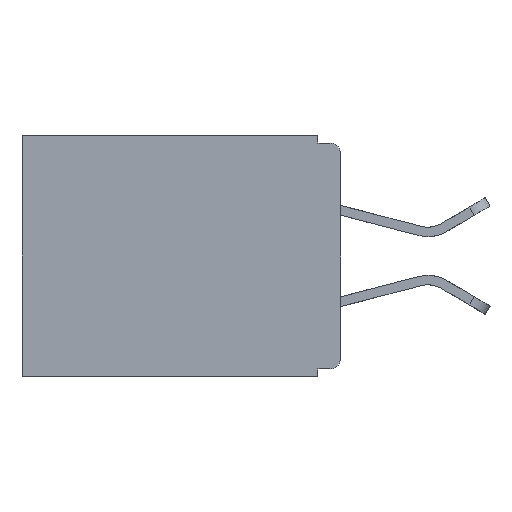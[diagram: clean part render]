
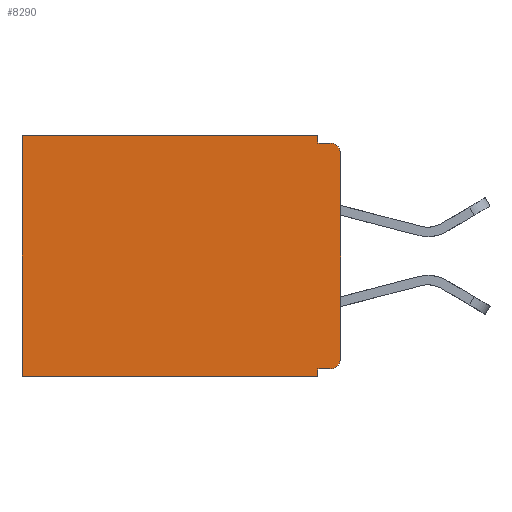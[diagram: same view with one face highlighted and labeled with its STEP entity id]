
A CAD part, left-side view. The second image highlights one B-rep face of the part: STEP entity #8290.
In plain terms, the highlighted planar face has unit normal (-1, 0, 0).
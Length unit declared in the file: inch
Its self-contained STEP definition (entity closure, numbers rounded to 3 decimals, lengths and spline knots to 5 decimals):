
#379 = LINE ( 'NONE', #2377, #12914 ) ;
#465 = DIRECTION ( 'NONE',  ( 0., 1., 0. ) ) ;
#565 = FACE_OUTER_BOUND ( 'NONE', #2653, .T. ) ;
#1374 = DIRECTION ( 'NONE',  ( 0., 1., 0. ) ) ;
#1641 = CARTESIAN_POINT ( 'NONE',  ( 0.3, 0.015, -0.025 ) ) ;
#1654 = EDGE_CURVE ( 'NONE', #6887, #11623, #3900, .T. ) ;
#2012 = DIRECTION ( 'NONE',  ( 0., -1., 0. ) ) ;
#2308 = ORIENTED_EDGE ( 'NONE', *, *, #12823, .F. ) ;
#2377 = CARTESIAN_POINT ( 'NONE',  ( 0.3, 0., 0. ) ) ;
#2424 = VECTOR ( 'NONE', #465, 39.37008 ) ;
#2498 = VECTOR ( 'NONE', #2619, 39.37008 ) ;
#2550 = VECTOR ( 'NONE', #4968, 39.37008 ) ;
#2619 = DIRECTION ( 'NONE',  ( 0., 0., -1. ) ) ;
#2653 = EDGE_LOOP ( 'NONE', ( #6909, #8642, #14633, #6433, #13592, #9976, #10757, #4682, #2308, #5501 ) ) ;
#2909 = DIRECTION ( 'NONE',  ( 0., 0., -1. ) ) ;
#2999 = EDGE_CURVE ( 'NONE', #15290, #11478, #9119, .T. ) ;
#3027 = CARTESIAN_POINT ( 'NONE',  ( 0.3, 0., -0.32 ) ) ;
#3900 = LINE ( 'NONE', #7316, #13713 ) ;
#4428 = VECTOR ( 'NONE', #2012, 39.37008 ) ;
#4554 = CARTESIAN_POINT ( 'NONE',  ( 0.3, 0.015, -0.305 ) ) ;
#4575 = DIRECTION ( 'NONE',  ( 0., 0., -1. ) ) ;
#4682 = ORIENTED_EDGE ( 'NONE', *, *, #1654, .F. ) ;
#4968 = DIRECTION ( 'NONE',  ( 0., 0., -1. ) ) ;
#5361 = CARTESIAN_POINT ( 'NONE',  ( 0.3, 0.031, -0.01 ) ) ;
#5400 = VERTEX_POINT ( 'NONE', #9719 ) ;
#5501 = ORIENTED_EDGE ( 'NONE', *, *, #12935, .T. ) ;
#5579 = CARTESIAN_POINT ( 'NONE',  ( 0.3, 0.031, 0. ) ) ;
#5631 = EDGE_CURVE ( 'NONE', #11623, #5400, #9064, .T. ) ;
#5797 = DIRECTION ( 'NONE',  ( 0., 0., -1. ) ) ;
#5834 = VECTOR ( 'NONE', #1374, 39.37008 ) ;
#6073 = CARTESIAN_POINT ( 'NONE',  ( 0.3, 0., -0.305 ) ) ;
#6237 = CARTESIAN_POINT ( 'NONE',  ( 0.3, 0.437, -0.33 ) ) ;
#6433 = ORIENTED_EDGE ( 'NONE', *, *, #2999, .F. ) ;
#6880 = EDGE_CURVE ( 'NONE', #11478, #10705, #10846, .T. ) ;
#6887 = VERTEX_POINT ( 'NONE', #11490 ) ;
#6909 = ORIENTED_EDGE ( 'NONE', *, *, #10507, .F. ) ;
#6969 = AXIS2_PLACEMENT_3D ( 'NONE', #1641, #10267, #2909 ) ;
#7316 = CARTESIAN_POINT ( 'NONE',  ( 0.3, 0.031, -0.33 ) ) ;
#7367 = CIRCLE ( 'NONE', #6969, 0.015 ) ;
#7947 = CIRCLE ( 'NONE', #13935, 0.015 ) ;
#8290 = ADVANCED_FACE ( 'NONE', ( #565 ), #9404, .F. ) ;
#8642 = ORIENTED_EDGE ( 'NONE', *, *, #12745, .T. ) ;
#8721 = EDGE_CURVE ( 'NONE', #15290, #11842, #379, .T. ) ;
#8919 = CARTESIAN_POINT ( 'NONE',  ( 0.3, 0.031, 0. ) ) ;
#9064 = LINE ( 'NONE', #9918, #5834 ) ;
#9119 = LINE ( 'NONE', #5579, #2498 ) ;
#9149 = DIRECTION ( 'NONE',  ( 0., 0., -1. ) ) ;
#9361 = DIRECTION ( 'NONE',  ( 1., 0., 0. ) ) ;
#9404 = PLANE ( 'NONE',  #14623 ) ;
#9686 = LINE ( 'NONE', #13874, #12013 ) ;
#9719 = CARTESIAN_POINT ( 'NONE',  ( 0.3, 0.437, -0.33 ) ) ;
#9765 = CARTESIAN_POINT ( 'NONE',  ( 0.3, 0., -0.33 ) ) ;
#9918 = CARTESIAN_POINT ( 'NONE',  ( 0.3, 0., -0.33 ) ) ;
#9962 = DIRECTION ( 'NONE',  ( 0., 0., -1. ) ) ;
#9976 = ORIENTED_EDGE ( 'NONE', *, *, #15141, .T. ) ;
#10267 = DIRECTION ( 'NONE',  ( -1., 0., 0. ) ) ;
#10507 = EDGE_CURVE ( 'NONE', #10637, #11201, #9686, .T. ) ;
#10617 = VERTEX_POINT ( 'NONE', #11923 ) ;
#10637 = VERTEX_POINT ( 'NONE', #15239 ) ;
#10705 = VERTEX_POINT ( 'NONE', #10988 ) ;
#10757 = ORIENTED_EDGE ( 'NONE', *, *, #5631, .F. ) ;
#10846 = LINE ( 'NONE', #12681, #4428 ) ;
#10988 = CARTESIAN_POINT ( 'NONE',  ( 0.3, 0.015, -0.01 ) ) ;
#11201 = VERTEX_POINT ( 'NONE', #6073 ) ;
#11413 = DIRECTION ( 'NONE',  ( 0., 1., 0. ) ) ;
#11478 = VERTEX_POINT ( 'NONE', #5361 ) ;
#11490 = CARTESIAN_POINT ( 'NONE',  ( 0.3, 0.031, -0.32 ) ) ;
#11623 = VERTEX_POINT ( 'NONE', #12618 ) ;
#11842 = VERTEX_POINT ( 'NONE', #15210 ) ;
#11923 = CARTESIAN_POINT ( 'NONE',  ( 0.3, 0.015, -0.32 ) ) ;
#12013 = VECTOR ( 'NONE', #4575, 39.37008 ) ;
#12618 = CARTESIAN_POINT ( 'NONE',  ( 0.3, 0.031, -0.33 ) ) ;
#12681 = CARTESIAN_POINT ( 'NONE',  ( 0.3, 0., -0.01 ) ) ;
#12745 = EDGE_CURVE ( 'NONE', #10637, #10705, #7367, .T. ) ;
#12822 = DIRECTION ( 'NONE',  ( -1., 0., 0. ) ) ;
#12823 = EDGE_CURVE ( 'NONE', #10617, #6887, #15033, .T. ) ;
#12914 = VECTOR ( 'NONE', #11413, 39.37008 ) ;
#12935 = EDGE_CURVE ( 'NONE', #10617, #11201, #7947, .T. ) ;
#13592 = ORIENTED_EDGE ( 'NONE', *, *, #8721, .T. ) ;
#13713 = VECTOR ( 'NONE', #9962, 39.37008 ) ;
#13874 = CARTESIAN_POINT ( 'NONE',  ( 0.3, 0., -0.33 ) ) ;
#13935 = AXIS2_PLACEMENT_3D ( 'NONE', #4554, #12822, #5797 ) ;
#14623 = AXIS2_PLACEMENT_3D ( 'NONE', #9765, #9361, #9149 ) ;
#14633 = ORIENTED_EDGE ( 'NONE', *, *, #6880, .F. ) ;
#15033 = LINE ( 'NONE', #3027, #2424 ) ;
#15123 = LINE ( 'NONE', #6237, #2550 ) ;
#15141 = EDGE_CURVE ( 'NONE', #11842, #5400, #15123, .T. ) ;
#15210 = CARTESIAN_POINT ( 'NONE',  ( 0.3, 0.437, 0. ) ) ;
#15239 = CARTESIAN_POINT ( 'NONE',  ( 0.3, 0., -0.025 ) ) ;
#15290 = VERTEX_POINT ( 'NONE', #8919 ) ;
